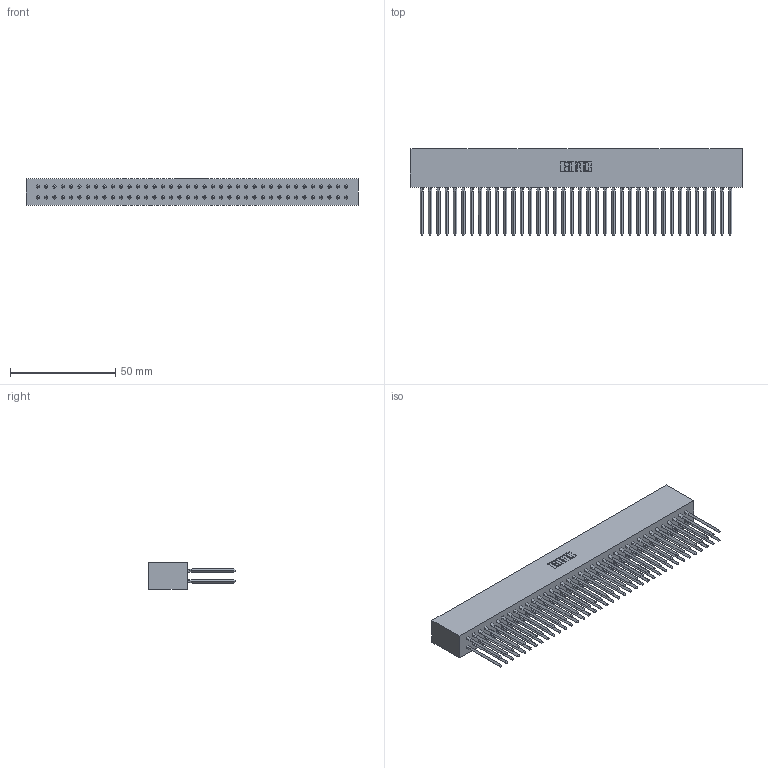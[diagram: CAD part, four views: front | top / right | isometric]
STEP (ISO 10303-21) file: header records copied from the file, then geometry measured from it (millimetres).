
FILE_DESCRIPTION (( 'STEP AP203' ), '1' );
FILE_NAME ('317-076-543-801.STEP', '2020-02-28T08:29:14', ( '' ), ( '' ), 'SwSTEP 2.0', 'SolidWorks 2016', '' );
FILE_SCHEMA (( 'CONFIG_CONTROL_DESIGN' ));
Length unit declared in the file: inch
Products named in the file (3): 317 Part_Lugless; 317-290-001_543; 317-076-543-801
Assembly tree (77 placements, depth 2):
  317-076-543-801
    317 Part_Lugless
    317-290-001_543  x76
Bounding box: 157.78 x 41.15 x 12.7 mm (x, y, z)
Volume: 28517.8 mm3; surface area: 43383 mm2
Topology: 77 solids, 77 shells, 6854 faces, 19011 edges, 12242 vertices
Faces by surface type: plane 5598, cylinder 952, bspline 304
Entity records: 55078 total; most frequent: CARTESIAN_POINT 10023, ORIENTED_EDGE 9522, DIRECTION 7935, EDGE_CURVE 4761, LINE 4513, VECTOR 4513, VERTEX_POINT 3167, AXIS2_PLACEMENT_3D 1711
